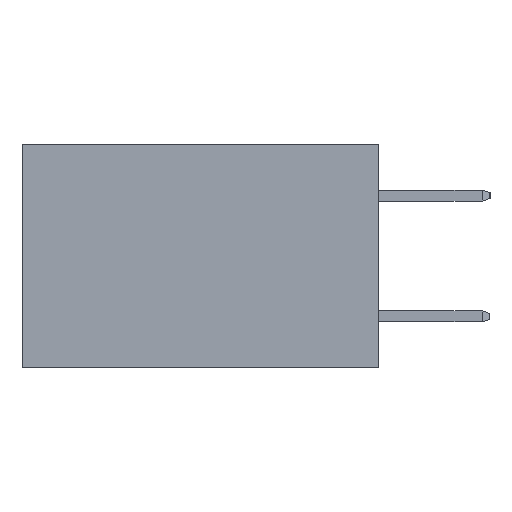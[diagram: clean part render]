
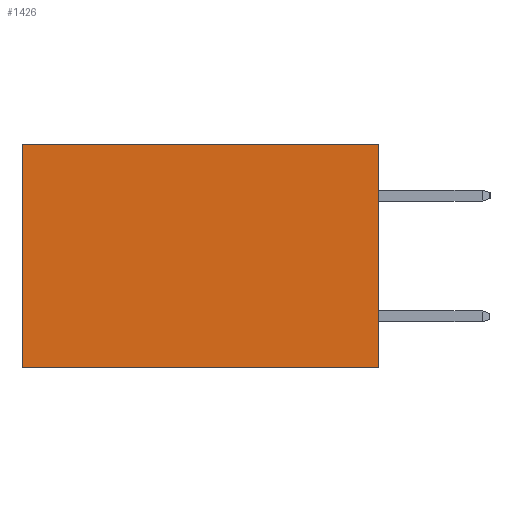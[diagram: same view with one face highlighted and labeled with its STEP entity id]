
A CAD part, left-side view. The second image highlights one B-rep face of the part: STEP entity #1426.
In plain terms, the highlighted planar face has unit normal (-1, 0, 0).
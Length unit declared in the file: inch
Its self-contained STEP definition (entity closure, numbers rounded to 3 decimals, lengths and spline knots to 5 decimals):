
#1426 = ADVANCED_FACE ( 'NONE', ( #2383 ), #14209, .F. ) ;
#2383 = FACE_OUTER_BOUND ( 'NONE', #6655, .T. ) ;
#3063 = ORIENTED_EDGE ( 'NONE', *, *, #18205, .T. ) ;
#3195 = LINE ( 'NONE', #10764, #10747 ) ;
#3480 = VECTOR ( 'NONE', #18220, 39.37008 ) ;
#4306 = CARTESIAN_POINT ( 'NONE',  ( 0.277, 0., 0. ) ) ;
#6261 = CARTESIAN_POINT ( 'NONE',  ( 0.277, 0., 0. ) ) ;
#6655 = EDGE_LOOP ( 'NONE', ( #10613, #6881, #19731, #3063 ) ) ;
#6881 = ORIENTED_EDGE ( 'NONE', *, *, #20614, .F. ) ;
#7262 = VERTEX_POINT ( 'NONE', #4306 ) ;
#7460 = CARTESIAN_POINT ( 'NONE',  ( 0.277, 0., -0.37 ) ) ;
#9379 = LINE ( 'NONE', #6261, #13145 ) ;
#9994 = DIRECTION ( 'NONE',  ( 0., 0., -1. ) ) ;
#10613 = ORIENTED_EDGE ( 'NONE', *, *, #20301, .T. ) ;
#10747 = VECTOR ( 'NONE', #20388, 39.37008 ) ;
#10764 = CARTESIAN_POINT ( 'NONE',  ( 0.277, 0., -0.37 ) ) ;
#11739 = VERTEX_POINT ( 'NONE', #12604 ) ;
#11842 = CARTESIAN_POINT ( 'NONE',  ( 0.277, 0., -0.37 ) ) ;
#12604 = CARTESIAN_POINT ( 'NONE',  ( 0.277, 0.59, -0.37 ) ) ;
#13145 = VECTOR ( 'NONE', #17597, 39.37008 ) ;
#13325 = CARTESIAN_POINT ( 'NONE',  ( 0.277, 0.59, -0.37 ) ) ;
#13918 = DIRECTION ( 'NONE',  ( 0., 0., -1. ) ) ;
#14209 = PLANE ( 'NONE',  #15631 ) ;
#14493 = CARTESIAN_POINT ( 'NONE',  ( 0.277, 0., -0.37 ) ) ;
#15493 = DIRECTION ( 'NONE',  ( 1., 0., 0. ) ) ;
#15631 = AXIS2_PLACEMENT_3D ( 'NONE', #14493, #15493, #9994 ) ;
#16283 = EDGE_CURVE ( 'NONE', #7262, #16758, #18623, .T. ) ;
#16596 = CARTESIAN_POINT ( 'NONE',  ( 0.277, 0.59, 0. ) ) ;
#16698 = VERTEX_POINT ( 'NONE', #16596 ) ;
#16758 = VERTEX_POINT ( 'NONE', #11842 ) ;
#16774 = VECTOR ( 'NONE', #13918, 39.37008 ) ;
#17369 = LINE ( 'NONE', #13325, #3480 ) ;
#17597 = DIRECTION ( 'NONE',  ( 0., 1., 0. ) ) ;
#18205 = EDGE_CURVE ( 'NONE', #7262, #16698, #9379, .T. ) ;
#18220 = DIRECTION ( 'NONE',  ( 0., 0., -1. ) ) ;
#18623 = LINE ( 'NONE', #7460, #16774 ) ;
#19731 = ORIENTED_EDGE ( 'NONE', *, *, #16283, .F. ) ;
#20301 = EDGE_CURVE ( 'NONE', #16698, #11739, #17369, .T. ) ;
#20388 = DIRECTION ( 'NONE',  ( 0., 1., 0. ) ) ;
#20614 = EDGE_CURVE ( 'NONE', #16758, #11739, #3195, .T. ) ;
